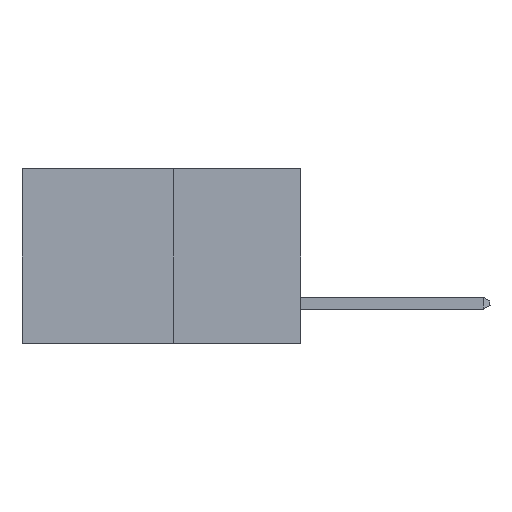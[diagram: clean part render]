
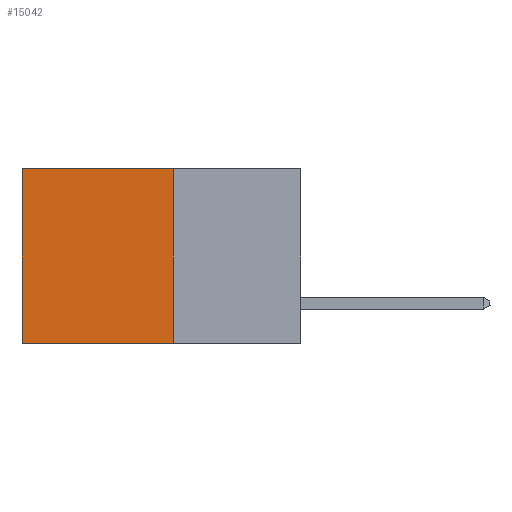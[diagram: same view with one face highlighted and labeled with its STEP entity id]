
A CAD part, left-side view. The second image highlights one B-rep face of the part: STEP entity #15042.
In plain terms, the highlighted planar face has unit normal (-1, 0, 0).
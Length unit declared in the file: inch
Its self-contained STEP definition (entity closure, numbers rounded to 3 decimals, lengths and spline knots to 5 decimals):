
#521 = ORIENTED_EDGE ( 'NONE', *, *, #4740, .T. ) ;
#1248 = VERTEX_POINT ( 'NONE', #5243 ) ;
#1976 = VECTOR ( 'NONE', #11728, 39.37008 ) ;
#2678 = EDGE_LOOP ( 'NONE', ( #20373, #21181, #20693, #521 ) ) ;
#2868 = CARTESIAN_POINT ( 'NONE',  ( 0.277, 0.27, -0.37 ) ) ;
#4740 = EDGE_CURVE ( 'NONE', #1248, #23324, #10120, .T. ) ;
#5243 = CARTESIAN_POINT ( 'NONE',  ( 0.277, 0.27, 0. ) ) ;
#6878 = LINE ( 'NONE', #18992, #1976 ) ;
#7110 = VERTEX_POINT ( 'NONE', #2868 ) ;
#8712 = CARTESIAN_POINT ( 'NONE',  ( 0.277, 0.27, -0.37 ) ) ;
#9168 = CARTESIAN_POINT ( 'NONE',  ( 0.277, 0.27, -0.37 ) ) ;
#10120 = LINE ( 'NONE', #22033, #15547 ) ;
#11150 = DIRECTION ( 'NONE',  ( 0., 1., 0. ) ) ;
#11728 = DIRECTION ( 'NONE',  ( 0., 1., 0. ) ) ;
#11803 = AXIS2_PLACEMENT_3D ( 'NONE', #8712, #23249, #12384 ) ;
#12249 = EDGE_CURVE ( 'NONE', #7110, #17120, #6878, .T. ) ;
#12384 = DIRECTION ( 'NONE',  ( 0., 0., -1. ) ) ;
#12422 = LINE ( 'NONE', #16054, #21499 ) ;
#12838 = LINE ( 'NONE', #9168, #17132 ) ;
#12919 = CARTESIAN_POINT ( 'NONE',  ( 0.277, 0.59, -0.37 ) ) ;
#13241 = EDGE_CURVE ( 'NONE', #1248, #7110, #12838, .T. ) ;
#15042 = ADVANCED_FACE ( 'NONE', ( #23229 ), #19630, .F. ) ;
#15547 = VECTOR ( 'NONE', #11150, 39.37008 ) ;
#16054 = CARTESIAN_POINT ( 'NONE',  ( 0.277, 0.59, -0.37 ) ) ;
#16511 = DIRECTION ( 'NONE',  ( 0., 0., -1. ) ) ;
#17120 = VERTEX_POINT ( 'NONE', #12919 ) ;
#17132 = VECTOR ( 'NONE', #16511, 39.37008 ) ;
#17892 = DIRECTION ( 'NONE',  ( 0., 0., -1. ) ) ;
#17969 = CARTESIAN_POINT ( 'NONE',  ( 0.277, 0.59, 0. ) ) ;
#18992 = CARTESIAN_POINT ( 'NONE',  ( 0.277, 0.27, -0.37 ) ) ;
#19630 = PLANE ( 'NONE',  #11803 ) ;
#20373 = ORIENTED_EDGE ( 'NONE', *, *, #23293, .T. ) ;
#20693 = ORIENTED_EDGE ( 'NONE', *, *, #13241, .F. ) ;
#21181 = ORIENTED_EDGE ( 'NONE', *, *, #12249, .F. ) ;
#21499 = VECTOR ( 'NONE', #17892, 39.37008 ) ;
#22033 = CARTESIAN_POINT ( 'NONE',  ( 0.277, 0.27, 0. ) ) ;
#23229 = FACE_OUTER_BOUND ( 'NONE', #2678, .T. ) ;
#23249 = DIRECTION ( 'NONE',  ( 1., 0., 0. ) ) ;
#23293 = EDGE_CURVE ( 'NONE', #23324, #17120, #12422, .T. ) ;
#23324 = VERTEX_POINT ( 'NONE', #17969 ) ;
